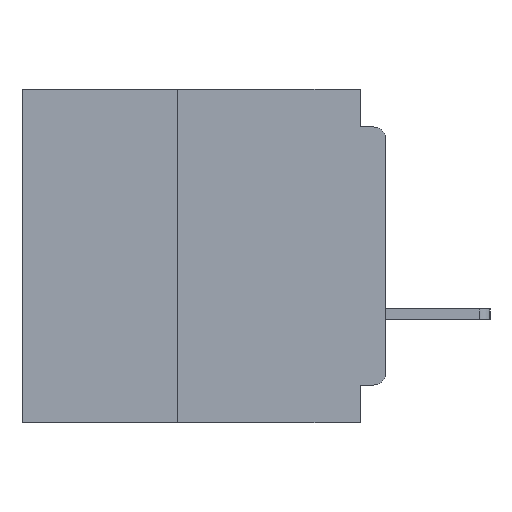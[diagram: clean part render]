
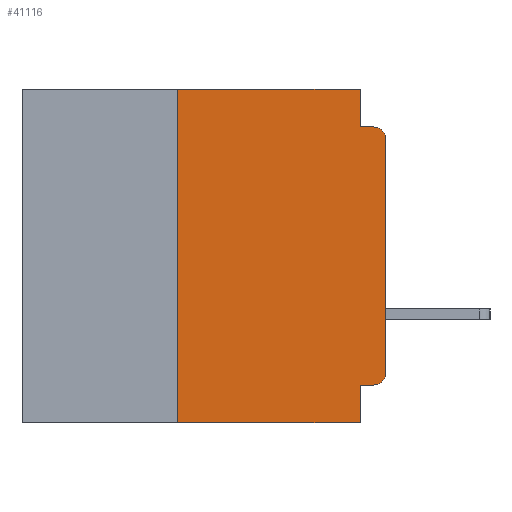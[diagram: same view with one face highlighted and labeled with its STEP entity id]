
A CAD part, left-side view. The second image highlights one B-rep face of the part: STEP entity #41116.
In plain terms, the highlighted planar face has unit normal (-1, 0, 0).
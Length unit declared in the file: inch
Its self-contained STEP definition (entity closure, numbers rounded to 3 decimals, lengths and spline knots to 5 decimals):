
#312 = AXIS2_PLACEMENT_3D ( 'NONE', #31886, #7537, #35929 ) ;
#789 = VERTEX_POINT ( 'NONE', #47270 ) ;
#1662 = VECTOR ( 'NONE', #46325, 39.37008 ) ;
#2650 = LINE ( 'NONE', #37254, #24513 ) ;
#2746 = CIRCLE ( 'NONE', #6756, 0.015 ) ;
#2942 = LINE ( 'NONE', #5740, #1662 ) ;
#2958 = CARTESIAN_POINT ( 'NONE',  ( 0., 0., -0.045 ) ) ;
#3980 = CARTESIAN_POINT ( 'NONE',  ( 0., 0., -0.355 ) ) ;
#4528 = CARTESIAN_POINT ( 'NONE',  ( 0., 0.031, -0.045 ) ) ;
#4733 = DIRECTION ( 'NONE',  ( 0., 0., -1. ) ) ;
#4888 = DIRECTION ( 'NONE',  ( 0., 0., 1. ) ) ;
#5740 = CARTESIAN_POINT ( 'NONE',  ( 0., 0.031, 0. ) ) ;
#6189 = DIRECTION ( 'NONE',  ( 1., 0., 0. ) ) ;
#6756 = AXIS2_PLACEMENT_3D ( 'NONE', #16640, #44741, #20709 ) ;
#6774 = VERTEX_POINT ( 'NONE', #25863 ) ;
#7537 = DIRECTION ( 'NONE',  ( -1., 0., 0. ) ) ;
#7709 = CARTESIAN_POINT ( 'NONE',  ( 0., 0.015, -0.045 ) ) ;
#7726 = EDGE_LOOP ( 'NONE', ( #17476, #18989, #19436, #20880, #21516, #22546, #23199, #28760, #34779, #35313 ) ) ;
#8777 = EDGE_CURVE ( 'NONE', #45386, #25952, #8867, .T. ) ;
#8867 = LINE ( 'NONE', #2958, #50571 ) ;
#10230 = PLANE ( 'NONE',  #25934 ) ;
#16640 = CARTESIAN_POINT ( 'NONE',  ( 0., 0.015, -0.06 ) ) ;
#17079 = FACE_OUTER_BOUND ( 'NONE', #7726, .T. ) ;
#17371 = CARTESIAN_POINT ( 'NONE',  ( 0., 0.25, -0.4 ) ) ;
#17476 = ORIENTED_EDGE ( 'NONE', *, *, #41310, .T. ) ;
#18989 = ORIENTED_EDGE ( 'NONE', *, *, #28821, .T. ) ;
#19436 = ORIENTED_EDGE ( 'NONE', *, *, #8777, .F. ) ;
#19842 = CARTESIAN_POINT ( 'NONE',  ( 0., 0., 0. ) ) ;
#20687 = LINE ( 'NONE', #17371, #40782 ) ;
#20709 = DIRECTION ( 'NONE',  ( 0., 0., -1. ) ) ;
#20880 = ORIENTED_EDGE ( 'NONE', *, *, #51974, .F. ) ;
#21103 = CARTESIAN_POINT ( 'NONE',  ( 0., 0.031, -0.4 ) ) ;
#21516 = ORIENTED_EDGE ( 'NONE', *, *, #30074, .F. ) ;
#22546 = ORIENTED_EDGE ( 'NONE', *, *, #49276, .F. ) ;
#23199 = ORIENTED_EDGE ( 'NONE', *, *, #35843, .T. ) ;
#23503 = EDGE_CURVE ( 'NONE', #42886, #44663, #40919, .T. ) ;
#23602 = CARTESIAN_POINT ( 'NONE',  ( 0., 0.031, 0. ) ) ;
#23912 = DIRECTION ( 'NONE',  ( 0., 0., 1. ) ) ;
#24102 = VERTEX_POINT ( 'NONE', #23602 ) ;
#24513 = VECTOR ( 'NONE', #45156, 39.37008 ) ;
#24540 = VECTOR ( 'NONE', #32513, 39.37008 ) ;
#25863 = CARTESIAN_POINT ( 'NONE',  ( 0., 0.25, -0.4 ) ) ;
#25934 = AXIS2_PLACEMENT_3D ( 'NONE', #30581, #6189, #34657 ) ;
#25952 = VERTEX_POINT ( 'NONE', #7709 ) ;
#26420 = VECTOR ( 'NONE', #44624, 39.37008 ) ;
#28760 = ORIENTED_EDGE ( 'NONE', *, *, #33175, .F. ) ;
#28821 = EDGE_CURVE ( 'NONE', #789, #25952, #2746, .T. ) ;
#30074 = EDGE_CURVE ( 'NONE', #30963, #24102, #47766, .T. ) ;
#30581 = CARTESIAN_POINT ( 'NONE',  ( 0., 0.437, 0. ) ) ;
#30908 = LINE ( 'NONE', #19842, #39074 ) ;
#30963 = VERTEX_POINT ( 'NONE', #50126 ) ;
#31517 = DIRECTION ( 'NONE',  ( 0., -1., 0. ) ) ;
#31886 = CARTESIAN_POINT ( 'NONE',  ( 0., 0.015, -0.34 ) ) ;
#31916 = CARTESIAN_POINT ( 'NONE',  ( 0., 0.015, -0.355 ) ) ;
#32513 = DIRECTION ( 'NONE',  ( 0., 1., 0. ) ) ;
#33175 = EDGE_CURVE ( 'NONE', #39743, #51858, #44799, .T. ) ;
#34657 = DIRECTION ( 'NONE',  ( 0., 0., -1. ) ) ;
#34779 = ORIENTED_EDGE ( 'NONE', *, *, #42339, .F. ) ;
#35313 = ORIENTED_EDGE ( 'NONE', *, *, #23503, .T. ) ;
#35843 = EDGE_CURVE ( 'NONE', #6774, #51858, #2650, .T. ) ;
#35929 = DIRECTION ( 'NONE',  ( 0., 0., -1. ) ) ;
#37254 = CARTESIAN_POINT ( 'NONE',  ( 0., 0.437, -0.4 ) ) ;
#37587 = CARTESIAN_POINT ( 'NONE',  ( 0., 0.031, -0.355 ) ) ;
#39074 = VECTOR ( 'NONE', #23912, 39.37008 ) ;
#39743 = VERTEX_POINT ( 'NONE', #37587 ) ;
#40349 = CARTESIAN_POINT ( 'NONE',  ( 0., 0., -0.34 ) ) ;
#40595 = CARTESIAN_POINT ( 'NONE',  ( 0., 0.437, 0. ) ) ;
#40782 = VECTOR ( 'NONE', #4888, 39.37008 ) ;
#40919 = CIRCLE ( 'NONE', #312, 0.015 ) ;
#41116 = ADVANCED_FACE ( 'NONE', ( #17079 ), #10230, .F. ) ;
#41310 = EDGE_CURVE ( 'NONE', #44663, #789, #30908, .T. ) ;
#41556 = CARTESIAN_POINT ( 'NONE',  ( 0., 0.031, -0.4 ) ) ;
#42339 = EDGE_CURVE ( 'NONE', #42886, #39743, #44600, .T. ) ;
#42886 = VERTEX_POINT ( 'NONE', #31916 ) ;
#43538 = VECTOR ( 'NONE', #4733, 39.37008 ) ;
#44600 = LINE ( 'NONE', #3980, #24540 ) ;
#44624 = DIRECTION ( 'NONE',  ( 0., -1., 0. ) ) ;
#44663 = VERTEX_POINT ( 'NONE', #40349 ) ;
#44741 = DIRECTION ( 'NONE',  ( -1., 0., 0. ) ) ;
#44799 = LINE ( 'NONE', #21103, #43538 ) ;
#45156 = DIRECTION ( 'NONE',  ( 0., -1., 0. ) ) ;
#45386 = VERTEX_POINT ( 'NONE', #4528 ) ;
#46325 = DIRECTION ( 'NONE',  ( 0., 0., -1. ) ) ;
#47270 = CARTESIAN_POINT ( 'NONE',  ( 0., 0., -0.06 ) ) ;
#47766 = LINE ( 'NONE', #40595, #26420 ) ;
#49276 = EDGE_CURVE ( 'NONE', #6774, #30963, #20687, .T. ) ;
#50126 = CARTESIAN_POINT ( 'NONE',  ( 0., 0.25, 0. ) ) ;
#50571 = VECTOR ( 'NONE', #31517, 39.37008 ) ;
#51858 = VERTEX_POINT ( 'NONE', #41556 ) ;
#51974 = EDGE_CURVE ( 'NONE', #24102, #45386, #2942, .T. ) ;
